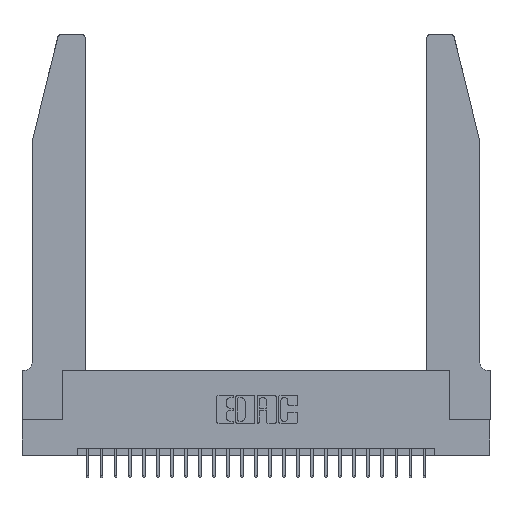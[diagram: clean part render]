
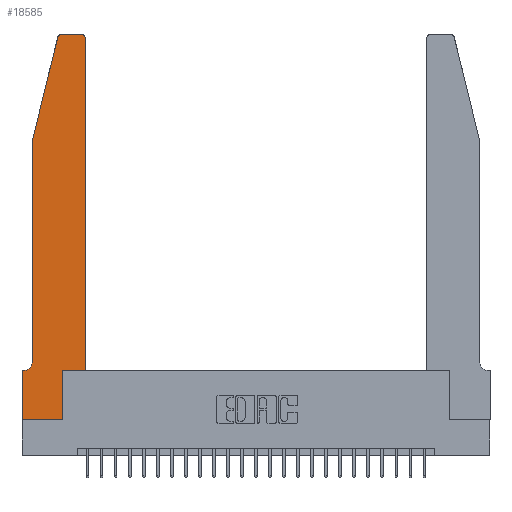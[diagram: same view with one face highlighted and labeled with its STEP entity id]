
A CAD part, top view. The second image highlights one B-rep face of the part: STEP entity #18585.
In plain terms, the highlighted planar face has unit normal (0, 0, 1).
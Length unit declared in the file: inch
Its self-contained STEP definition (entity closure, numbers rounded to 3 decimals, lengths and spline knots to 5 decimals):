
#25 = DIRECTION ( 'NONE',  ( 1., 0., 0. ) ) ;
#260 = ORIENTED_EDGE ( 'NONE', *, *, #18141, .T. ) ;
#577 = CARTESIAN_POINT ( 'NONE',  ( 0.4505, 0.35, 0.37 ) ) ;
#665 = AXIS2_PLACEMENT_3D ( 'NONE', #9087, #12756, #17519 ) ;
#1012 = VERTEX_POINT ( 'NONE', #15957 ) ;
#1330 = VECTOR ( 'NONE', #13300, 39.37008 ) ;
#1910 = EDGE_CURVE ( 'NONE', #22745, #23519, #3824, .T. ) ;
#2058 = VERTEX_POINT ( 'NONE', #8561 ) ;
#2540 = VECTOR ( 'NONE', #9620, 39.37008 ) ;
#2936 = ORIENTED_EDGE ( 'NONE', *, *, #23264, .T. ) ;
#3086 = VERTEX_POINT ( 'NONE', #25921 ) ;
#3824 = CIRCLE ( 'NONE', #16685, 0.03 ) ;
#3842 = VERTEX_POINT ( 'NONE', #8771 ) ;
#3878 = CARTESIAN_POINT ( 'NONE',  ( 0.2865, 0.35, 0.37 ) ) ;
#3993 = CARTESIAN_POINT ( 'NONE',  ( 0., 0., 0.37 ) ) ;
#4297 = LINE ( 'NONE', #3878, #15905 ) ;
#5008 = EDGE_CURVE ( 'NONE', #2058, #18790, #11722, .T. ) ;
#5198 = VERTEX_POINT ( 'NONE', #20713 ) ;
#5302 = ORIENTED_EDGE ( 'NONE', *, *, #9569, .T. ) ;
#6042 = DIRECTION ( 'NONE',  ( -1., 0., 0. ) ) ;
#6341 = DIRECTION ( 'NONE',  ( 0., 0., 1. ) ) ;
#6735 = DIRECTION ( 'NONE',  ( 0., 0., 1. ) ) ;
#6841 = LINE ( 'NONE', #26680, #14540 ) ;
#6896 = LINE ( 'NONE', #25683, #1330 ) ;
#7042 = VECTOR ( 'NONE', #19231, 39.37008 ) ;
#7242 = LINE ( 'NONE', #12161, #26588 ) ;
#7380 = CARTESIAN_POINT ( 'NONE',  ( 0.4205, 2.75, 0.37 ) ) ;
#7760 = LINE ( 'NONE', #22467, #16735 ) ;
#8232 = ORIENTED_EDGE ( 'NONE', *, *, #5008, .T. ) ;
#8559 = CIRCLE ( 'NONE', #665, 0.03 ) ;
#8561 = CARTESIAN_POINT ( 'NONE',  ( 0.2865, 0.35, 0.37 ) ) ;
#8591 = EDGE_CURVE ( 'NONE', #18790, #25280, #9205, .T. ) ;
#8771 = CARTESIAN_POINT ( 'NONE',  ( 0., 0.35, 0.37 ) ) ;
#9087 = CARTESIAN_POINT ( 'NONE',  ( 0.4205, 2.72, 0.37 ) ) ;
#9205 = LINE ( 'NONE', #14007, #22088 ) ;
#9569 = EDGE_CURVE ( 'NONE', #3086, #2058, #4297, .T. ) ;
#9620 = DIRECTION ( 'NONE',  ( -1., 0., 0. ) ) ;
#10338 = CIRCLE ( 'NONE', #23327, 0.07 ) ;
#10834 = ORIENTED_EDGE ( 'NONE', *, *, #8591, .T. ) ;
#11722 = LINE ( 'NONE', #577, #26237 ) ;
#12161 = CARTESIAN_POINT ( 'NONE',  ( 0., 0., 0.37 ) ) ;
#12265 = CARTESIAN_POINT ( 'NONE',  ( 0.284, 2.72, 0.37 ) ) ;
#12422 = EDGE_CURVE ( 'NONE', #14753, #22745, #16125, .T. ) ;
#12574 = DIRECTION ( 'NONE',  ( 1., 0., 0. ) ) ;
#12616 = EDGE_CURVE ( 'NONE', #5198, #17288, #7760, .T. ) ;
#12736 = PLANE ( 'NONE',  #13421 ) ;
#12756 = DIRECTION ( 'NONE',  ( 0., 0., 1. ) ) ;
#12995 = EDGE_CURVE ( 'NONE', #17288, #1012, #10338, .T. ) ;
#13300 = DIRECTION ( 'NONE',  ( 0., -1., 0. ) ) ;
#13375 = CARTESIAN_POINT ( 'NONE',  ( 0.4505, 2.72, 0.37 ) ) ;
#13421 = AXIS2_PLACEMENT_3D ( 'NONE', #18852, #6735, #12574 ) ;
#13443 = ORIENTED_EDGE ( 'NONE', *, *, #20104, .T. ) ;
#14007 = CARTESIAN_POINT ( 'NONE',  ( 0.4505, 0.35, 0.37 ) ) ;
#14367 = CARTESIAN_POINT ( 'NONE',  ( 0.0055, 0.42, 0.37 ) ) ;
#14428 = LINE ( 'NONE', #21314, #7042 ) ;
#14540 = VECTOR ( 'NONE', #22519, 39.37008 ) ;
#14753 = VERTEX_POINT ( 'NONE', #7380 ) ;
#15522 = EDGE_CURVE ( 'NONE', #16118, #3086, #7242, .T. ) ;
#15783 = FACE_OUTER_BOUND ( 'NONE', #16862, .T. ) ;
#15905 = VECTOR ( 'NONE', #20439, 39.37008 ) ;
#15957 = CARTESIAN_POINT ( 'NONE',  ( 0.0055, 0.35, 0.37 ) ) ;
#16118 = VERTEX_POINT ( 'NONE', #3993 ) ;
#16125 = LINE ( 'NONE', #20210, #2540 ) ;
#16525 = CARTESIAN_POINT ( 'NONE',  ( 0.25487, 2.72718, 0.37 ) ) ;
#16685 = AXIS2_PLACEMENT_3D ( 'NONE', #12265, #6341, #20442 ) ;
#16735 = VECTOR ( 'NONE', #24637, 39.37008 ) ;
#16862 = EDGE_LOOP ( 'NONE', ( #24491, #17031, #13443, #19289, #23062, #260, #19512, #20937, #5302, #8232, #10834, #2936 ) ) ;
#17031 = ORIENTED_EDGE ( 'NONE', *, *, #1910, .T. ) ;
#17288 = VERTEX_POINT ( 'NONE', #18268 ) ;
#17519 = DIRECTION ( 'NONE',  ( 1., 0., 0. ) ) ;
#18141 = EDGE_CURVE ( 'NONE', #1012, #3842, #6841, .T. ) ;
#18206 = CARTESIAN_POINT ( 'NONE',  ( 0.284, 2.75, 0.37 ) ) ;
#18268 = CARTESIAN_POINT ( 'NONE',  ( 0.0755, 0.42, 0.37 ) ) ;
#18520 = CARTESIAN_POINT ( 'NONE',  ( 0.4505, 0.35, 0.37 ) ) ;
#18585 = ADVANCED_FACE ( 'NONE', ( #15783 ), #12736, .T. ) ;
#18790 = VERTEX_POINT ( 'NONE', #18520 ) ;
#18852 = CARTESIAN_POINT ( 'NONE',  ( 0., 0.35, 0.37 ) ) ;
#19231 = DIRECTION ( 'NONE',  ( -0.239, -0.971, 0. ) ) ;
#19289 = ORIENTED_EDGE ( 'NONE', *, *, #12616, .T. ) ;
#19512 = ORIENTED_EDGE ( 'NONE', *, *, #24577, .T. ) ;
#20104 = EDGE_CURVE ( 'NONE', #23519, #5198, #14428, .T. ) ;
#20210 = CARTESIAN_POINT ( 'NONE',  ( 0.2605, 2.75, 0.37 ) ) ;
#20439 = DIRECTION ( 'NONE',  ( 0., 1., 0. ) ) ;
#20442 = DIRECTION ( 'NONE',  ( 1., 0., 0. ) ) ;
#20713 = CARTESIAN_POINT ( 'NONE',  ( 0.0755, 2., 0.37 ) ) ;
#20937 = ORIENTED_EDGE ( 'NONE', *, *, #15522, .T. ) ;
#21253 = DIRECTION ( 'NONE',  ( 1., 0., 0. ) ) ;
#21314 = CARTESIAN_POINT ( 'NONE',  ( 0.0755, 2., 0.37 ) ) ;
#22088 = VECTOR ( 'NONE', #23186, 39.37008 ) ;
#22467 = CARTESIAN_POINT ( 'NONE',  ( 0.0755, 2., 0.37 ) ) ;
#22519 = DIRECTION ( 'NONE',  ( -1., 0., 0. ) ) ;
#22745 = VERTEX_POINT ( 'NONE', #18206 ) ;
#23062 = ORIENTED_EDGE ( 'NONE', *, *, #12995, .T. ) ;
#23186 = DIRECTION ( 'NONE',  ( 0., 1., 0. ) ) ;
#23264 = EDGE_CURVE ( 'NONE', #25280, #14753, #8559, .T. ) ;
#23327 = AXIS2_PLACEMENT_3D ( 'NONE', #14367, #26660, #6042 ) ;
#23519 = VERTEX_POINT ( 'NONE', #16525 ) ;
#24491 = ORIENTED_EDGE ( 'NONE', *, *, #12422, .T. ) ;
#24577 = EDGE_CURVE ( 'NONE', #3842, #16118, #6896, .T. ) ;
#24637 = DIRECTION ( 'NONE',  ( 0., -1., 0. ) ) ;
#25280 = VERTEX_POINT ( 'NONE', #13375 ) ;
#25683 = CARTESIAN_POINT ( 'NONE',  ( 0., 0., 0.37 ) ) ;
#25921 = CARTESIAN_POINT ( 'NONE',  ( 0.2865, 0., 0.37 ) ) ;
#26237 = VECTOR ( 'NONE', #21253, 39.37008 ) ;
#26588 = VECTOR ( 'NONE', #25, 39.37008 ) ;
#26660 = DIRECTION ( 'NONE',  ( 0., 0., -1. ) ) ;
#26680 = CARTESIAN_POINT ( 'NONE',  ( 0.0755, 0.35, 0.37 ) ) ;
